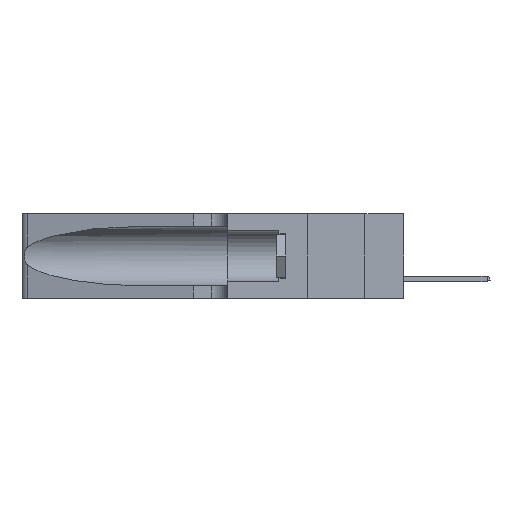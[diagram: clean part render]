
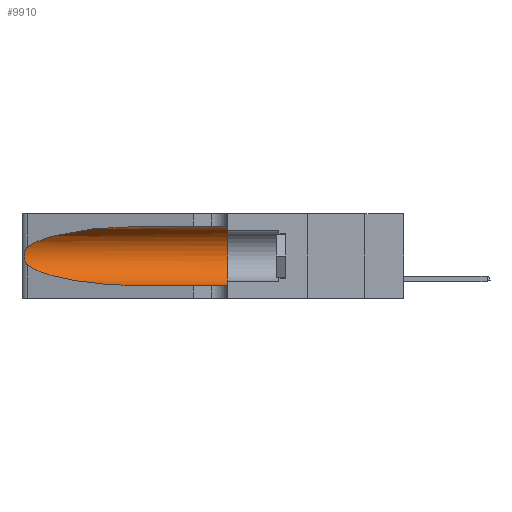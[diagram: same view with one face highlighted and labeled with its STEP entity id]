
A CAD part, left-side view. The second image highlights one B-rep face of the part: STEP entity #9910.
In plain terms, the highlighted cylindrical face has radius 3.308 mm (diameter 6.617 mm), a partial arc.
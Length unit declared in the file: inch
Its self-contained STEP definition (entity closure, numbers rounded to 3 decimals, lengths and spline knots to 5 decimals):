
#51 = CARTESIAN_POINT ( 'NONE',  ( 0.25854, 1.2359, 0.20912 ) ) ;
#138 = CARTESIAN_POINT ( 'NONE',  ( 0.25487, 1.22718, 0.14631 ) ) ;
#1068 = AXIS2_PLACEMENT_3D ( 'NONE', #8638, #23157, #10767 ) ;
#1428 = ORIENTED_EDGE ( 'NONE', *, *, #14014, .T. ) ;
#1678 = CARTESIAN_POINT ( 'NONE',  ( 0.1305, 1.61858, 0.05475 ) ) ;
#1850 = CARTESIAN_POINT ( 'NONE',  ( 0.1305, 0.72297, 0.05475 ) ) ;
#2263 = CARTESIAN_POINT ( 'NONE',  ( 0.25639, 1.23186, 0.15144 ) ) ;
#2350 = VERTEX_POINT ( 'NONE', #2572 ) ;
#2458 = VERTEX_POINT ( 'NONE', #24187 ) ;
#2572 = CARTESIAN_POINT ( 'NONE',  ( 0.1305, 0.35, 0.31525 ) ) ;
#2631 = CARTESIAN_POINT ( 'NONE',  ( 0.25789, 1.23486, 0.15765 ) ) ;
#2762 = CARTESIAN_POINT ( 'NONE',  ( 0.1305, 1.61858, 0.185 ) ) ;
#2899 =( BOUNDED_CURVE ( )  B_SPLINE_CURVE ( 3, ( #15860, #24310, #20153, #24758 ),
 .UNSPECIFIED., .F., .F. ) 
 B_SPLINE_CURVE_WITH_KNOTS ( ( 4, 4 ),
 ( 3.44316, 4.71239 ),
 .UNSPECIFIED. ) 
 CURVE ( )  GEOMETRIC_REPRESENTATION_ITEM ( )  RATIONAL_B_SPLINE_CURVE ( ( 1., 0.87, 0.87, 1. ) ) 
 REPRESENTATION_ITEM ( '' )  );
#4149 = CARTESIAN_POINT ( 'NONE',  ( 0.25639, 1.23184, 0.21858 ) ) ;
#5552 = DIRECTION ( 'NONE',  ( 0., -1., 0. ) ) ;
#6036 = CYLINDRICAL_SURFACE ( 'NONE', #26989, 0.13025 ) ;
#6213 = EDGE_CURVE ( 'NONE', #8192, #2350, #23126, .T. ) ;
#6426 = CARTESIAN_POINT ( 'NONE',  ( 0.25555, 1.22993, 0.14849 ) ) ;
#6539 = ORIENTED_EDGE ( 'NONE', *, *, #10983, .F. ) ;
#6757 = ORIENTED_EDGE ( 'NONE', *, *, #21292, .T. ) ;
#7410 =( BOUNDED_CURVE ( )  B_SPLINE_CURVE ( 3, ( #22261, #22453, #24288, #22349 ),
 .UNSPECIFIED., .F., .F. ) 
 B_SPLINE_CURVE_WITH_KNOTS ( ( 4, 4 ),
 ( 1.5708, 2.84003 ),
 .UNSPECIFIED. ) 
 CURVE ( )  GEOMETRIC_REPRESENTATION_ITEM ( )  RATIONAL_B_SPLINE_CURVE ( ( 1., 0.87, 0.87, 1. ) ) 
 REPRESENTATION_ITEM ( '' )  );
#7582 = EDGE_LOOP ( 'NONE', ( #14239, #6757, #1428, #10958, #6539, #7879 ) ) ;
#7879 = ORIENTED_EDGE ( 'NONE', *, *, #6213, .F. ) ;
#8192 = VERTEX_POINT ( 'NONE', #24963 ) ;
#8571 = VECTOR ( 'NONE', #5552, 39.37008 ) ;
#8638 = CARTESIAN_POINT ( 'NONE',  ( 0.1305, 0.35, 0.185 ) ) ;
#8909 = CARTESIAN_POINT ( 'NONE',  ( 0.26075, 1.23896, 0.178 ) ) ;
#9910 = ADVANCED_FACE ( 'NONE', ( #16837 ), #6036, .F. ) ;
#9983 = EDGE_CURVE ( 'NONE', #8192, #2458, #7410, .T. ) ;
#10551 = CARTESIAN_POINT ( 'NONE',  ( 0.26018, 1.23835, 0.19895 ) ) ;
#10767 = DIRECTION ( 'NONE',  ( 0., 0., 1. ) ) ;
#10958 = ORIENTED_EDGE ( 'NONE', *, *, #11693, .T. ) ;
#10983 = EDGE_CURVE ( 'NONE', #2350, #13303, #26733, .T. ) ;
#11693 = EDGE_CURVE ( 'NONE', #22789, #13303, #15826, .T. ) ;
#11871 = CARTESIAN_POINT ( 'NONE',  ( 0.1305, 1.61858, 0.31525 ) ) ;
#13303 = VERTEX_POINT ( 'NONE', #19409 ) ;
#14014 = EDGE_CURVE ( 'NONE', #14502, #22789, #2899, .T. ) ;
#14239 = ORIENTED_EDGE ( 'NONE', *, *, #9983, .T. ) ;
#14500 = CARTESIAN_POINT ( 'NONE',  ( 0.25487, 1.22718, 0.22369 ) ) ;
#14502 = VERTEX_POINT ( 'NONE', #25038 ) ;
#14591 = CARTESIAN_POINT ( 'NONE',  ( 0.25555, 1.22994, 0.2215 ) ) ;
#14672 = CARTESIAN_POINT ( 'NONE',  ( 0.26075, 1.23896, 0.19203 ) ) ;
#15361 = DIRECTION ( 'NONE',  ( 0., -1., 0. ) ) ;
#15826 = LINE ( 'NONE', #1678, #8571 ) ;
#15860 = CARTESIAN_POINT ( 'NONE',  ( 0.25487, 1.22718, 0.14631 ) ) ;
#16837 = FACE_OUTER_BOUND ( 'NONE', #7582, .T. ) ;
#17138 = CARTESIAN_POINT ( 'NONE',  ( 0.25856, 1.23593, 0.16098 ) ) ;
#17511 = VECTOR ( 'NONE', #22158, 39.37008 ) ;
#18793 = CARTESIAN_POINT ( 'NONE',  ( 0.25787, 1.23484, 0.2124 ) ) ;
#19409 = CARTESIAN_POINT ( 'NONE',  ( 0.1305, 0.35, 0.05475 ) ) ;
#20153 = CARTESIAN_POINT ( 'NONE',  ( 0.18966, 0.96281, 0.05475 ) ) ;
#21292 = EDGE_CURVE ( 'NONE', #2458, #14502, #22042, .T. ) ;
#21366 = CARTESIAN_POINT ( 'NONE',  ( 0.26017, 1.23833, 0.17102 ) ) ;
#22042 = B_SPLINE_CURVE_WITH_KNOTS ( 'NONE', 3,
 ( #14500, #14591, #4149, #18793, #51, #10551, #14672, #8909, #21366, #17138, #2631, #2263, #6426, #138 ),
 .UNSPECIFIED., .F., .F.,
 ( 4, 2, 2, 2, 2, 2, 4 ),
 ( 0., 0.00027, 0.00053, 0.00107, 0.0016, 0.00187, 0.00214 ),
 .UNSPECIFIED. ) ;
#22158 = DIRECTION ( 'NONE',  ( 0., -1., 0. ) ) ;
#22261 = CARTESIAN_POINT ( 'NONE',  ( 0.1305, 0.72297, 0.31525 ) ) ;
#22349 = CARTESIAN_POINT ( 'NONE',  ( 0.25487, 1.22718, 0.22369 ) ) ;
#22453 = CARTESIAN_POINT ( 'NONE',  ( 0.18966, 0.96281, 0.31525 ) ) ;
#22789 = VERTEX_POINT ( 'NONE', #1850 ) ;
#23126 = LINE ( 'NONE', #11871, #17511 ) ;
#23157 = DIRECTION ( 'NONE',  ( 0., 1., 0. ) ) ;
#24187 = CARTESIAN_POINT ( 'NONE',  ( 0.25487, 1.22718, 0.22369 ) ) ;
#24288 = CARTESIAN_POINT ( 'NONE',  ( 0.2373, 1.15595, 0.28018 ) ) ;
#24310 = CARTESIAN_POINT ( 'NONE',  ( 0.2373, 1.15595, 0.08982 ) ) ;
#24758 = CARTESIAN_POINT ( 'NONE',  ( 0.1305, 0.72297, 0.05475 ) ) ;
#24963 = CARTESIAN_POINT ( 'NONE',  ( 0.1305, 0.72297, 0.31525 ) ) ;
#25038 = CARTESIAN_POINT ( 'NONE',  ( 0.25487, 1.22718, 0.14631 ) ) ;
#26121 = DIRECTION ( 'NONE',  ( 0., 0., -1. ) ) ;
#26733 = CIRCLE ( 'NONE', #1068, 0.13025 ) ;
#26989 = AXIS2_PLACEMENT_3D ( 'NONE', #2762, #15361, #26121 ) ;
